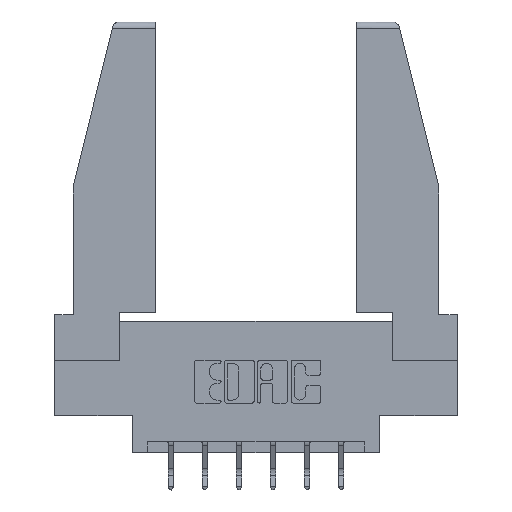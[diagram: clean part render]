
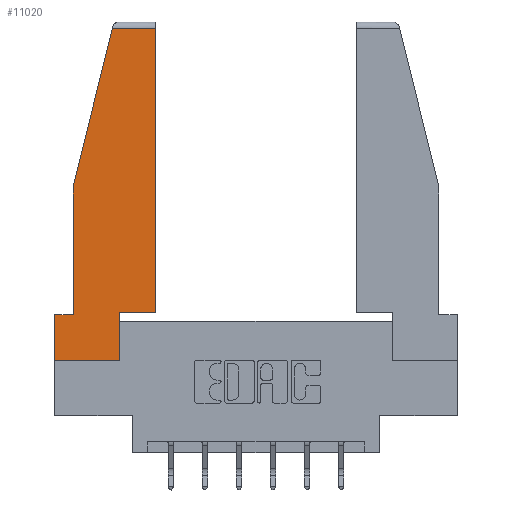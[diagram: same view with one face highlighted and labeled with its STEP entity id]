
A CAD part, top view. The second image highlights one B-rep face of the part: STEP entity #11020.
In plain terms, the highlighted planar face has unit normal (0, 0, 1).
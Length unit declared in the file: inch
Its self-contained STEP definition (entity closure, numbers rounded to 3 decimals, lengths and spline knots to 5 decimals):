
#22 = VECTOR ( 'NONE', #9634, 39.37008 ) ;
#381 = VERTEX_POINT ( 'NONE', #2942 ) ;
#888 = ORIENTED_EDGE ( 'NONE', *, *, #7597, .T. ) ;
#1143 = CARTESIAN_POINT ( 'NONE',  ( 0., 0.21, 0. ) ) ;
#1229 = CARTESIAN_POINT ( 'NONE',  ( 0.297, 0., 0. ) ) ;
#1299 = CARTESIAN_POINT ( 'NONE',  ( 0., 0., 0. ) ) ;
#1432 = EDGE_CURVE ( 'NONE', #3557, #5604, #7767, .T. ) ;
#1614 = EDGE_CURVE ( 'NONE', #11442, #381, #11307, .T. ) ;
#2022 = CARTESIAN_POINT ( 'NONE',  ( 0., 0.21, 0. ) ) ;
#2068 = DIRECTION ( 'NONE',  ( -1., 0., 0. ) ) ;
#2224 = CARTESIAN_POINT ( 'NONE',  ( 0.297, 0., 0. ) ) ;
#2397 = CARTESIAN_POINT ( 'NONE',  ( 0., 0., 0. ) ) ;
#2667 = ORIENTED_EDGE ( 'NONE', *, *, #1614, .T. ) ;
#2668 = CARTESIAN_POINT ( 'NONE',  ( 0.461, 0.223, 0. ) ) ;
#2711 = DIRECTION ( 'NONE',  ( 0., 1., 0. ) ) ;
#2758 = VERTEX_POINT ( 'NONE', #8747 ) ;
#2942 = CARTESIAN_POINT ( 'NONE',  ( 0.086, 0.21, 0. ) ) ;
#2959 = DIRECTION ( 'NONE',  ( -1., 0., 0. ) ) ;
#2979 = VECTOR ( 'NONE', #2959, 39.37008 ) ;
#3142 = VECTOR ( 'NONE', #3313, 39.37008 ) ;
#3313 = DIRECTION ( 'NONE',  ( 1., 0., 0. ) ) ;
#3349 = CARTESIAN_POINT ( 'NONE',  ( 0.461, 0.223, 0. ) ) ;
#3374 = DIRECTION ( 'NONE',  ( 1., 0., 0. ) ) ;
#3437 = LINE ( 'NONE', #2397, #3142 ) ;
#3513 = CARTESIAN_POINT ( 'NONE',  ( 0.461, 1.52, 0. ) ) ;
#3557 = VERTEX_POINT ( 'NONE', #2022 ) ;
#3682 = EDGE_CURVE ( 'NONE', #5103, #10190, #3952, .T. ) ;
#3833 = VECTOR ( 'NONE', #4221, 39.37008 ) ;
#3952 = LINE ( 'NONE', #4284, #11124 ) ;
#3969 = LINE ( 'NONE', #1229, #10680 ) ;
#3999 = CARTESIAN_POINT ( 'NONE',  ( 0., 1.52, 0. ) ) ;
#4180 = VERTEX_POINT ( 'NONE', #3513 ) ;
#4221 = DIRECTION ( 'NONE',  ( 0., -1., 0. ) ) ;
#4241 = ORIENTED_EDGE ( 'NONE', *, *, #6957, .T. ) ;
#4284 = CARTESIAN_POINT ( 'NONE',  ( 0.297, 0.223, 0. ) ) ;
#4605 = ORIENTED_EDGE ( 'NONE', *, *, #3682, .T. ) ;
#4808 = VECTOR ( 'NONE', #9515, 39.37008 ) ;
#4990 = EDGE_CURVE ( 'NONE', #381, #3557, #8378, .T. ) ;
#5015 = CARTESIAN_POINT ( 'NONE',  ( 0., 0., 0. ) ) ;
#5060 = AXIS2_PLACEMENT_3D ( 'NONE', #5015, #6195, #11554 ) ;
#5103 = VERTEX_POINT ( 'NONE', #11672 ) ;
#5600 = FACE_OUTER_BOUND ( 'NONE', #11213, .T. ) ;
#5604 = VERTEX_POINT ( 'NONE', #1299 ) ;
#5789 = VERTEX_POINT ( 'NONE', #2224 ) ;
#5818 = DIRECTION ( 'NONE',  ( 0., 1., 0. ) ) ;
#5849 = EDGE_CURVE ( 'NONE', #10190, #4180, #8932, .T. ) ;
#6195 = DIRECTION ( 'NONE',  ( 0., 0., 1. ) ) ;
#6957 = EDGE_CURVE ( 'NONE', #5789, #5103, #3969, .T. ) ;
#7368 = ORIENTED_EDGE ( 'NONE', *, *, #4990, .T. ) ;
#7597 = EDGE_CURVE ( 'NONE', #2758, #11442, #10661, .T. ) ;
#7767 = LINE ( 'NONE', #11285, #22 ) ;
#7781 = PLANE ( 'NONE',  #5060 ) ;
#7940 = LINE ( 'NONE', #3999, #2979 ) ;
#8378 = LINE ( 'NONE', #1143, #10219 ) ;
#8747 = CARTESIAN_POINT ( 'NONE',  ( 0.2636, 1.52, 0. ) ) ;
#8932 = LINE ( 'NONE', #2668, #11879 ) ;
#8946 = EDGE_CURVE ( 'NONE', #5604, #5789, #3437, .T. ) ;
#9279 = ORIENTED_EDGE ( 'NONE', *, *, #5849, .T. ) ;
#9515 = DIRECTION ( 'NONE',  ( -0.239, -0.971, 0. ) ) ;
#9634 = DIRECTION ( 'NONE',  ( 0., -1., 0. ) ) ;
#9789 = CARTESIAN_POINT ( 'NONE',  ( 0.086, 0.8, 0. ) ) ;
#10190 = VERTEX_POINT ( 'NONE', #3349 ) ;
#10219 = VECTOR ( 'NONE', #2068, 39.37008 ) ;
#10504 = ORIENTED_EDGE ( 'NONE', *, *, #1432, .T. ) ;
#10591 = ORIENTED_EDGE ( 'NONE', *, *, #10922, .T. ) ;
#10661 = LINE ( 'NONE', #11290, #4808 ) ;
#10680 = VECTOR ( 'NONE', #5818, 39.37008 ) ;
#10922 = EDGE_CURVE ( 'NONE', #4180, #2758, #7940, .T. ) ;
#11020 = ADVANCED_FACE ( 'NONE', ( #5600 ), #7781, .T. ) ;
#11059 = CARTESIAN_POINT ( 'NONE',  ( 0.086, 0.8, 0. ) ) ;
#11124 = VECTOR ( 'NONE', #3374, 39.37008 ) ;
#11213 = EDGE_LOOP ( 'NONE', ( #9279, #10591, #888, #2667, #7368, #10504, #11414, #4241, #4605 ) ) ;
#11285 = CARTESIAN_POINT ( 'NONE',  ( 0., 0.21, 0. ) ) ;
#11290 = CARTESIAN_POINT ( 'NONE',  ( 0.271, 1.55, 0. ) ) ;
#11307 = LINE ( 'NONE', #9789, #3833 ) ;
#11414 = ORIENTED_EDGE ( 'NONE', *, *, #8946, .T. ) ;
#11442 = VERTEX_POINT ( 'NONE', #11059 ) ;
#11554 = DIRECTION ( 'NONE',  ( 1., 0., 0. ) ) ;
#11672 = CARTESIAN_POINT ( 'NONE',  ( 0.297, 0.223, 0. ) ) ;
#11879 = VECTOR ( 'NONE', #2711, 39.37008 ) ;
